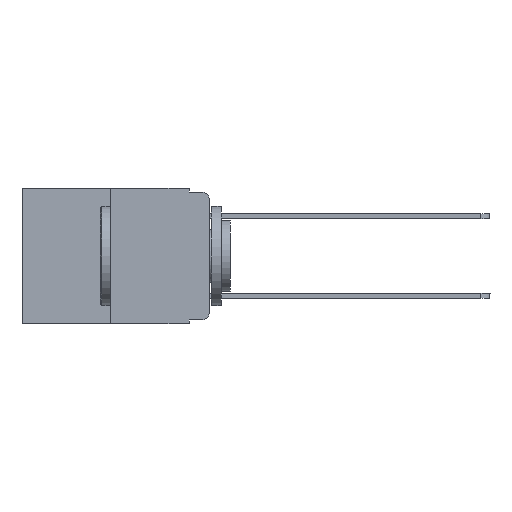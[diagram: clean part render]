
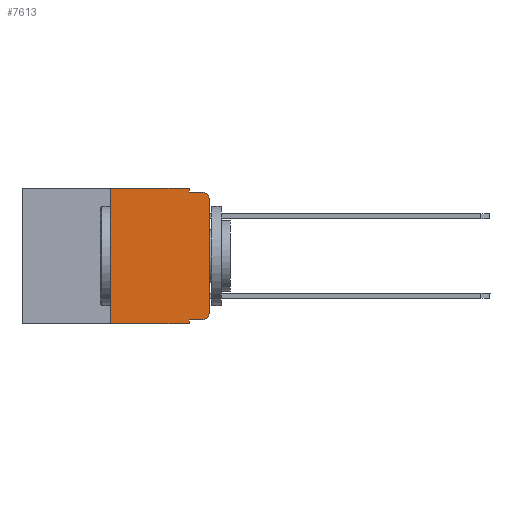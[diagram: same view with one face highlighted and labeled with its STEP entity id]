
A CAD part, left-side view. The second image highlights one B-rep face of the part: STEP entity #7613.
In plain terms, the highlighted planar face has unit normal (-1, 0, 0).
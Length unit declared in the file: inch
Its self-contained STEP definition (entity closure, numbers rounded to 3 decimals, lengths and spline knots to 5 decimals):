
#152 = LINE ( 'NONE', #10890, #2231 ) ;
#753 = CARTESIAN_POINT ( 'NONE',  ( 0., 0.051, 0. ) ) ;
#844 = VERTEX_POINT ( 'NONE', #8891 ) ;
#854 = CARTESIAN_POINT ( 'NONE',  ( 0., 0.02, -0.01 ) ) ;
#1092 = DIRECTION ( 'NONE',  ( 0., 0., -1. ) ) ;
#1241 = ORIENTED_EDGE ( 'NONE', *, *, #11857, .T. ) ;
#1258 = CARTESIAN_POINT ( 'NONE',  ( 0., 0., -0.313 ) ) ;
#1287 = VERTEX_POINT ( 'NONE', #854 ) ;
#1408 = LINE ( 'NONE', #8257, #10617 ) ;
#1554 = LINE ( 'NONE', #13888, #9461 ) ;
#1705 = DIRECTION ( 'NONE',  ( 0., 0., -1. ) ) ;
#2026 = DIRECTION ( 'NONE',  ( 0., -1., 0. ) ) ;
#2098 = LINE ( 'NONE', #15878, #13059 ) ;
#2216 = ORIENTED_EDGE ( 'NONE', *, *, #3267, .T. ) ;
#2231 = VECTOR ( 'NONE', #16454, 39.37008 ) ;
#2378 = VERTEX_POINT ( 'NONE', #5327 ) ;
#3196 = DIRECTION ( 'NONE',  ( 0., 0., -1. ) ) ;
#3267 = EDGE_CURVE ( 'NONE', #9293, #1287, #6341, .T. ) ;
#3356 = LINE ( 'NONE', #6378, #16172 ) ;
#4086 = CARTESIAN_POINT ( 'NONE',  ( 0., 0.02, -0.333 ) ) ;
#5130 = FACE_OUTER_BOUND ( 'NONE', #15360, .T. ) ;
#5313 = DIRECTION ( 'NONE',  ( 1., 0., 0. ) ) ;
#5327 = CARTESIAN_POINT ( 'NONE',  ( 0., 0.25, 0. ) ) ;
#5838 = EDGE_CURVE ( 'NONE', #844, #2378, #10882, .T. ) ;
#5879 = EDGE_CURVE ( 'NONE', #8077, #7292, #1408, .T. ) ;
#6278 = VECTOR ( 'NONE', #1705, 39.37008 ) ;
#6341 = CIRCLE ( 'NONE', #10935, 0.02 ) ;
#6378 = CARTESIAN_POINT ( 'NONE',  ( 0., 0.051, -0.01 ) ) ;
#6831 = EDGE_CURVE ( 'NONE', #17006, #14528, #9596, .T. ) ;
#7292 = VERTEX_POINT ( 'NONE', #7367 ) ;
#7367 = CARTESIAN_POINT ( 'NONE',  ( 0., 0.051, -0.343 ) ) ;
#7392 = AXIS2_PLACEMENT_3D ( 'NONE', #8244, #5313, #7982 ) ;
#7613 = ADVANCED_FACE ( 'NONE', ( #5130 ), #17707, .F. ) ;
#7675 = ORIENTED_EDGE ( 'NONE', *, *, #5838, .F. ) ;
#7896 = ORIENTED_EDGE ( 'NONE', *, *, #6831, .T. ) ;
#7982 = DIRECTION ( 'NONE',  ( 0., 0., -1. ) ) ;
#8077 = VERTEX_POINT ( 'NONE', #13624 ) ;
#8244 = CARTESIAN_POINT ( 'NONE',  ( 0., 0.473, 0. ) ) ;
#8257 = CARTESIAN_POINT ( 'NONE',  ( 0., 0.051, 0. ) ) ;
#8457 = DIRECTION ( 'NONE',  ( -1., 0., 0. ) ) ;
#8567 = EDGE_CURVE ( 'NONE', #13997, #9526, #8642, .T. ) ;
#8642 = LINE ( 'NONE', #13955, #6278 ) ;
#8891 = CARTESIAN_POINT ( 'NONE',  ( 0., 0.25, -0.343 ) ) ;
#8908 = ORIENTED_EDGE ( 'NONE', *, *, #10026, .T. ) ;
#9206 = DIRECTION ( 'NONE',  ( -1., 0., 0. ) ) ;
#9277 = ORIENTED_EDGE ( 'NONE', *, *, #8567, .F. ) ;
#9293 = VERTEX_POINT ( 'NONE', #13117 ) ;
#9300 = CARTESIAN_POINT ( 'NONE',  ( 0., 0.02, -0.03 ) ) ;
#9461 = VECTOR ( 'NONE', #15317, 39.37008 ) ;
#9526 = VERTEX_POINT ( 'NONE', #11318 ) ;
#9596 = CIRCLE ( 'NONE', #14195, 0.02 ) ;
#10026 = EDGE_CURVE ( 'NONE', #8077, #17006, #1554, .T. ) ;
#10068 = CARTESIAN_POINT ( 'NONE',  ( 0., 0.02, -0.313 ) ) ;
#10617 = VECTOR ( 'NONE', #13745, 39.37008 ) ;
#10882 = LINE ( 'NONE', #17443, #13476 ) ;
#10890 = CARTESIAN_POINT ( 'NONE',  ( 0., 0.473, 0. ) ) ;
#10935 = AXIS2_PLACEMENT_3D ( 'NONE', #9300, #9206, #1092 ) ;
#11254 = VECTOR ( 'NONE', #12879, 39.37008 ) ;
#11318 = CARTESIAN_POINT ( 'NONE',  ( 0., 0.051, -0.01 ) ) ;
#11459 = CARTESIAN_POINT ( 'NONE',  ( 0., 0.473, -0.343 ) ) ;
#11838 = DIRECTION ( 'NONE',  ( 0., 0., 1. ) ) ;
#11857 = EDGE_CURVE ( 'NONE', #844, #7292, #14407, .T. ) ;
#12443 = ORIENTED_EDGE ( 'NONE', *, *, #5879, .F. ) ;
#12879 = DIRECTION ( 'NONE',  ( 0., -1., 0. ) ) ;
#13059 = VECTOR ( 'NONE', #11838, 39.37008 ) ;
#13117 = CARTESIAN_POINT ( 'NONE',  ( 0., 0., -0.03 ) ) ;
#13476 = VECTOR ( 'NONE', #16357, 39.37008 ) ;
#13486 = EDGE_CURVE ( 'NONE', #9526, #1287, #3356, .T. ) ;
#13624 = CARTESIAN_POINT ( 'NONE',  ( 0., 0.051, -0.333 ) ) ;
#13745 = DIRECTION ( 'NONE',  ( 0., 0., -1. ) ) ;
#13888 = CARTESIAN_POINT ( 'NONE',  ( 0., 0.051, -0.333 ) ) ;
#13955 = CARTESIAN_POINT ( 'NONE',  ( 0., 0.051, 0. ) ) ;
#13997 = VERTEX_POINT ( 'NONE', #753 ) ;
#14195 = AXIS2_PLACEMENT_3D ( 'NONE', #10068, #8457, #3196 ) ;
#14407 = LINE ( 'NONE', #11459, #11254 ) ;
#14528 = VERTEX_POINT ( 'NONE', #1258 ) ;
#15012 = ORIENTED_EDGE ( 'NONE', *, *, #15327, .T. ) ;
#15317 = DIRECTION ( 'NONE',  ( 0., -1., 0. ) ) ;
#15327 = EDGE_CURVE ( 'NONE', #14528, #9293, #2098, .T. ) ;
#15360 = EDGE_LOOP ( 'NONE', ( #15012, #2216, #15969, #9277, #16479, #7675, #1241, #12443, #8908, #7896 ) ) ;
#15878 = CARTESIAN_POINT ( 'NONE',  ( 0., 0., 0. ) ) ;
#15969 = ORIENTED_EDGE ( 'NONE', *, *, #13486, .F. ) ;
#16172 = VECTOR ( 'NONE', #2026, 39.37008 ) ;
#16353 = EDGE_CURVE ( 'NONE', #2378, #13997, #152, .T. ) ;
#16357 = DIRECTION ( 'NONE',  ( 0., 0., 1. ) ) ;
#16454 = DIRECTION ( 'NONE',  ( 0., -1., 0. ) ) ;
#16479 = ORIENTED_EDGE ( 'NONE', *, *, #16353, .F. ) ;
#17006 = VERTEX_POINT ( 'NONE', #4086 ) ;
#17443 = CARTESIAN_POINT ( 'NONE',  ( 0., 0.25, 0. ) ) ;
#17707 = PLANE ( 'NONE',  #7392 ) ;
